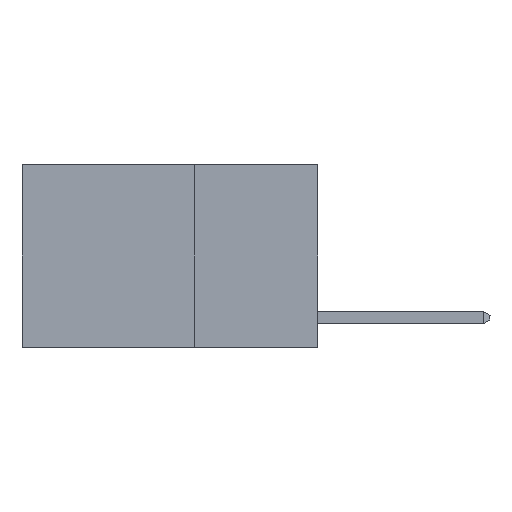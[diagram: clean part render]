
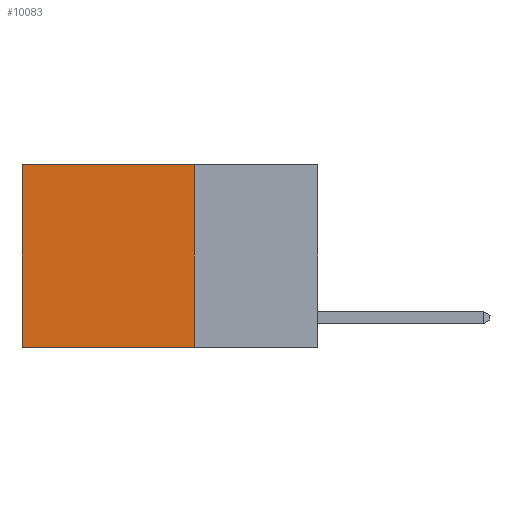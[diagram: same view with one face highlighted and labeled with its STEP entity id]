
A CAD part, left-side view. The second image highlights one B-rep face of the part: STEP entity #10083.
In plain terms, the highlighted planar face has unit normal (-1, 0, 0).
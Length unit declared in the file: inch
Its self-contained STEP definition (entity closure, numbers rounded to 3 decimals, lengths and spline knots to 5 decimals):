
#317 = CARTESIAN_POINT ( 'NONE',  ( 0.2625, 0.6, 0. ) ) ;
#1113 = LINE ( 'NONE', #6128, #20058 ) ;
#1373 = DIRECTION ( 'NONE',  ( 0., 0., -1. ) ) ;
#1706 = CARTESIAN_POINT ( 'NONE',  ( 0.2625, 0.6, 0. ) ) ;
#2074 = EDGE_CURVE ( 'NONE', #2480, #10020, #20109, .T. ) ;
#2480 = VERTEX_POINT ( 'NONE', #22678 ) ;
#2881 = VECTOR ( 'NONE', #20745, 39.37008 ) ;
#3274 = ORIENTED_EDGE ( 'NONE', *, *, #20454, .T. ) ;
#3296 = PLANE ( 'NONE',  #6330 ) ;
#6083 = ORIENTED_EDGE ( 'NONE', *, *, #10406, .T. ) ;
#6128 = CARTESIAN_POINT ( 'NONE',  ( 0.2625, 0.25, 0. ) ) ;
#6330 = AXIS2_PLACEMENT_3D ( 'NONE', #8914, #23829, #12662 ) ;
#6645 = CARTESIAN_POINT ( 'NONE',  ( 0.2625, 0.25, 0. ) ) ;
#7045 = ORIENTED_EDGE ( 'NONE', *, *, #21727, .F. ) ;
#7952 = CARTESIAN_POINT ( 'NONE',  ( 0.2625, 0.6, -0.37 ) ) ;
#8914 = CARTESIAN_POINT ( 'NONE',  ( 0.2625, 0.25, 0. ) ) ;
#10020 = VERTEX_POINT ( 'NONE', #7952 ) ;
#10083 = ADVANCED_FACE ( 'NONE', ( #10420 ), #3296, .F. ) ;
#10208 = VERTEX_POINT ( 'NONE', #1706 ) ;
#10406 = EDGE_CURVE ( 'NONE', #11451, #10208, #1113, .T. ) ;
#10420 = FACE_OUTER_BOUND ( 'NONE', #12644, .T. ) ;
#11451 = VERTEX_POINT ( 'NONE', #20279 ) ;
#12644 = EDGE_LOOP ( 'NONE', ( #3274, #12912, #7045, #6083 ) ) ;
#12662 = DIRECTION ( 'NONE',  ( 0., 0., -1. ) ) ;
#12912 = ORIENTED_EDGE ( 'NONE', *, *, #2074, .F. ) ;
#13997 = LINE ( 'NONE', #317, #17832 ) ;
#17340 = VECTOR ( 'NONE', #1373, 39.37008 ) ;
#17832 = VECTOR ( 'NONE', #20935, 39.37008 ) ;
#20058 = VECTOR ( 'NONE', #21082, 39.37008 ) ;
#20109 = LINE ( 'NONE', #21256, #2881 ) ;
#20279 = CARTESIAN_POINT ( 'NONE',  ( 0.2625, 0.25, 0. ) ) ;
#20454 = EDGE_CURVE ( 'NONE', #10208, #10020, #13997, .T. ) ;
#20745 = DIRECTION ( 'NONE',  ( 0., 1., 0. ) ) ;
#20935 = DIRECTION ( 'NONE',  ( 0., 0., -1. ) ) ;
#21082 = DIRECTION ( 'NONE',  ( 0., 1., 0. ) ) ;
#21256 = CARTESIAN_POINT ( 'NONE',  ( 0.2625, 0.25, -0.37 ) ) ;
#21677 = LINE ( 'NONE', #6645, #17340 ) ;
#21727 = EDGE_CURVE ( 'NONE', #11451, #2480, #21677, .T. ) ;
#22678 = CARTESIAN_POINT ( 'NONE',  ( 0.2625, 0.25, -0.37 ) ) ;
#23829 = DIRECTION ( 'NONE',  ( 1., 0., 0. ) ) ;
